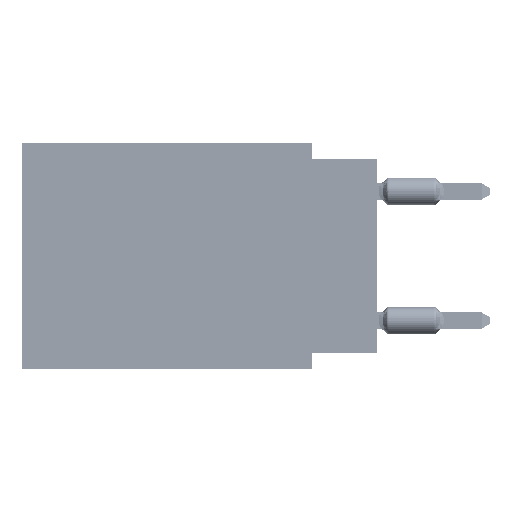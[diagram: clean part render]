
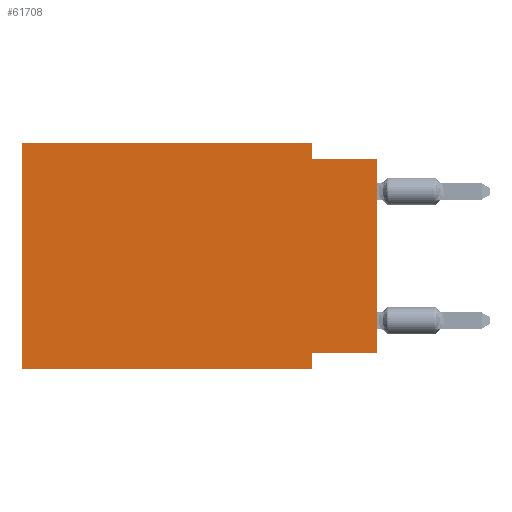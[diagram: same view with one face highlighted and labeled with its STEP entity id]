
A CAD part, left-side view. The second image highlights one B-rep face of the part: STEP entity #61708.
In plain terms, the highlighted planar face has unit normal (-1, 0, 0).
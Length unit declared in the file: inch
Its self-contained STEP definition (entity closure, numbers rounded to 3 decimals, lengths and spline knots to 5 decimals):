
#301 = CARTESIAN_POINT ( 'NONE',  ( 0., 0.55, 0. ) ) ;
#443 = LINE ( 'NONE', #79055, #49522 ) ;
#658 = DIRECTION ( 'NONE',  ( 0., 0., 1. ) ) ;
#1741 = ORIENTED_EDGE ( 'NONE', *, *, #18368, .F. ) ;
#4419 = EDGE_CURVE ( 'NONE', #65221, #13289, #43612, .T. ) ;
#8052 = DIRECTION ( 'NONE',  ( 0., 0., -1. ) ) ;
#9023 = CARTESIAN_POINT ( 'NONE',  ( 0., 0.1, 0. ) ) ;
#9833 = LINE ( 'NONE', #59011, #41857 ) ;
#11894 = EDGE_CURVE ( 'NONE', #30877, #48342, #22871, .T. ) ;
#12626 = CARTESIAN_POINT ( 'NONE',  ( 0., 0.1, -0.325 ) ) ;
#13213 = PLANE ( 'NONE',  #39243 ) ;
#13289 = VERTEX_POINT ( 'NONE', #54188 ) ;
#13639 = DIRECTION ( 'NONE',  ( 0., -1., 0. ) ) ;
#13856 = EDGE_CURVE ( 'NONE', #57755, #31467, #443, .T. ) ;
#18368 = EDGE_CURVE ( 'NONE', #57755, #37245, #51586, .T. ) ;
#19686 = DIRECTION ( 'NONE',  ( 1., 0., 0. ) ) ;
#22871 = LINE ( 'NONE', #77399, #54901 ) ;
#24896 = LINE ( 'NONE', #34811, #73980 ) ;
#25764 = VECTOR ( 'NONE', #51869, 39.37008 ) ;
#27568 = ORIENTED_EDGE ( 'NONE', *, *, #13856, .T. ) ;
#29598 = CARTESIAN_POINT ( 'NONE',  ( 0., 0., -0.325 ) ) ;
#30477 = ORIENTED_EDGE ( 'NONE', *, *, #51691, .F. ) ;
#30877 = VERTEX_POINT ( 'NONE', #49822 ) ;
#31084 = FACE_OUTER_BOUND ( 'NONE', #62596, .T. ) ;
#31467 = VERTEX_POINT ( 'NONE', #37746 ) ;
#34811 = CARTESIAN_POINT ( 'NONE',  ( 0., 0.55, -0.35 ) ) ;
#36302 = CARTESIAN_POINT ( 'NONE',  ( 0., 0.1, 0. ) ) ;
#36592 = VECTOR ( 'NONE', #37749, 39.37008 ) ;
#37245 = VERTEX_POINT ( 'NONE', #12626 ) ;
#37746 = CARTESIAN_POINT ( 'NONE',  ( 0., 0., -0.025 ) ) ;
#37749 = DIRECTION ( 'NONE',  ( 0., 1., 0. ) ) ;
#38414 = ORIENTED_EDGE ( 'NONE', *, *, #70298, .F. ) ;
#39010 = CARTESIAN_POINT ( 'NONE',  ( 0., 0., -0.025 ) ) ;
#39243 = AXIS2_PLACEMENT_3D ( 'NONE', #301, #19686, #64449 ) ;
#40295 = VECTOR ( 'NONE', #13639, 39.37008 ) ;
#40659 = DIRECTION ( 'NONE',  ( 0., 0., 1. ) ) ;
#41857 = VECTOR ( 'NONE', #8052, 39.37008 ) ;
#43612 = LINE ( 'NONE', #36302, #47657 ) ;
#47657 = VECTOR ( 'NONE', #74674, 39.37008 ) ;
#48215 = ORIENTED_EDGE ( 'NONE', *, *, #4419, .F. ) ;
#48342 = VERTEX_POINT ( 'NONE', #64840 ) ;
#49522 = VECTOR ( 'NONE', #40659, 39.37008 ) ;
#49822 = CARTESIAN_POINT ( 'NONE',  ( 0., 0.55, -0.35 ) ) ;
#51586 = LINE ( 'NONE', #69678, #36592 ) ;
#51691 = EDGE_CURVE ( 'NONE', #37245, #58048, #9833, .T. ) ;
#51869 = DIRECTION ( 'NONE',  ( 0., -1., 0. ) ) ;
#54188 = CARTESIAN_POINT ( 'NONE',  ( 0., 0.1, -0.025 ) ) ;
#54481 = EDGE_CURVE ( 'NONE', #48342, #65221, #57322, .T. ) ;
#54901 = VECTOR ( 'NONE', #658, 39.37008 ) ;
#57322 = LINE ( 'NONE', #77472, #40295 ) ;
#57755 = VERTEX_POINT ( 'NONE', #29598 ) ;
#58048 = VERTEX_POINT ( 'NONE', #58078 ) ;
#58078 = CARTESIAN_POINT ( 'NONE',  ( 0., 0.1, -0.35 ) ) ;
#59011 = CARTESIAN_POINT ( 'NONE',  ( 0., 0.1, -0.35 ) ) ;
#60531 = DIRECTION ( 'NONE',  ( 0., -1., 0. ) ) ;
#61708 = ADVANCED_FACE ( 'NONE', ( #31084 ), #13213, .F. ) ;
#62596 = EDGE_LOOP ( 'NONE', ( #27568, #38414, #48215, #76557, #64879, #75011, #30477, #1741 ) ) ;
#64449 = DIRECTION ( 'NONE',  ( 0., 0., -1. ) ) ;
#64840 = CARTESIAN_POINT ( 'NONE',  ( 0., 0.55, 0. ) ) ;
#64879 = ORIENTED_EDGE ( 'NONE', *, *, #11894, .F. ) ;
#65221 = VERTEX_POINT ( 'NONE', #9023 ) ;
#69678 = CARTESIAN_POINT ( 'NONE',  ( 0., 0., -0.325 ) ) ;
#70298 = EDGE_CURVE ( 'NONE', #13289, #31467, #76824, .T. ) ;
#73980 = VECTOR ( 'NONE', #60531, 39.37008 ) ;
#74674 = DIRECTION ( 'NONE',  ( 0., 0., -1. ) ) ;
#75011 = ORIENTED_EDGE ( 'NONE', *, *, #78309, .T. ) ;
#76557 = ORIENTED_EDGE ( 'NONE', *, *, #54481, .F. ) ;
#76824 = LINE ( 'NONE', #39010, #25764 ) ;
#77399 = CARTESIAN_POINT ( 'NONE',  ( 0., 0.55, 0. ) ) ;
#77472 = CARTESIAN_POINT ( 'NONE',  ( 0., 0.55, 0. ) ) ;
#78309 = EDGE_CURVE ( 'NONE', #30877, #58048, #24896, .T. ) ;
#79055 = CARTESIAN_POINT ( 'NONE',  ( 0., 0., 0. ) ) ;
